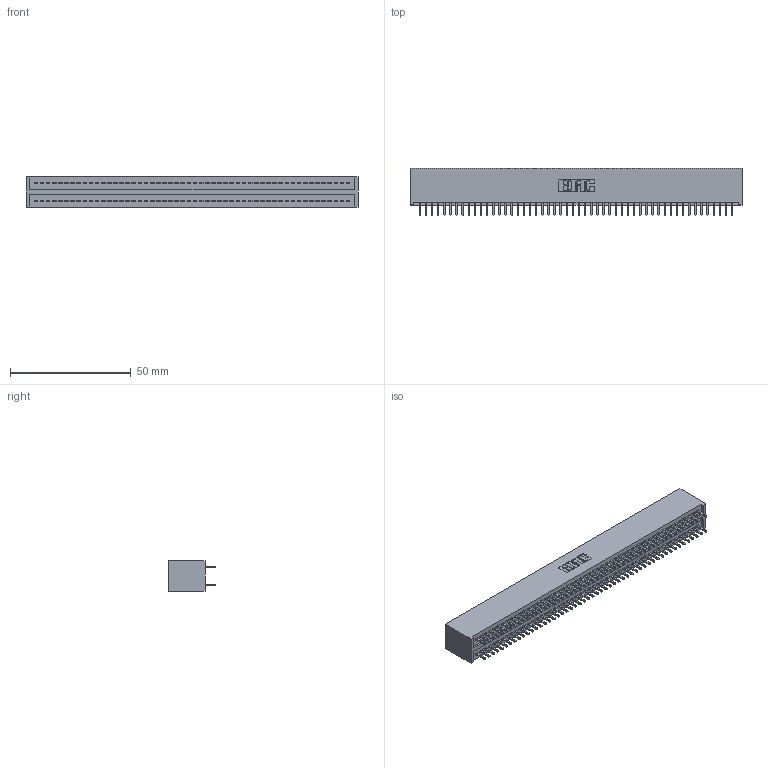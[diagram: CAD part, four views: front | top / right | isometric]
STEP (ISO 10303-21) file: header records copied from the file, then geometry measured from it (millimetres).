
FILE_DESCRIPTION (( 'STEP AP203' ), '1' );
FILE_NAME ('325-104-520-201.STEP', '2020-02-25T07:01:06', ( '' ), ( '' ), 'SwSTEP 2.0', 'SolidWorks 2016', '' );
FILE_SCHEMA (( 'CONFIG_CONTROL_DESIGN' ));
Length unit declared in the file: inch
Products named in the file (3): 325-104-520-201; 325 Part_Lugless; 325-292-001_325-293-120
Assembly tree (105 placements, depth 2):
  325-104-520-201
    325 Part_Lugless
    325-292-001_325-293-120  x104
Bounding box: 137.72 x 19.68 x 12.45 mm (x, y, z)
Volume: 18459.2 mm3; surface area: 23030.4 mm2
Topology: 105 solids, 105 shells, 5514 faces, 16407 edges, 10798 vertices
Faces by surface type: plane 3810, cylinder 1704
Entity records: 31901 total; most frequent: CARTESIAN_POINT 5274, ORIENTED_EDGE 5210, DIRECTION 4481, EDGE_CURVE 2605, LINE 2485, VECTOR 2485, VERTEX_POINT 1734, AXIS2_PLACEMENT_3D 998
